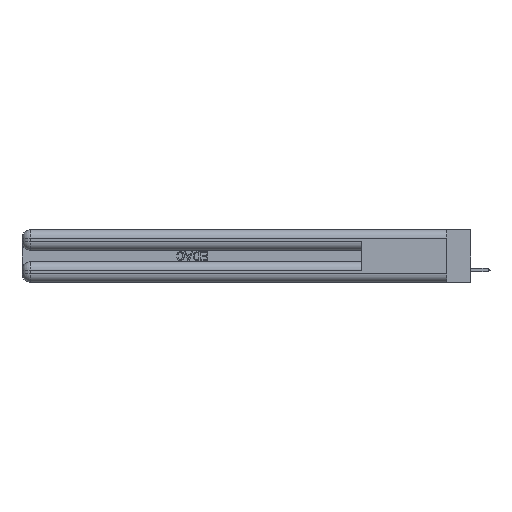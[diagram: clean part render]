
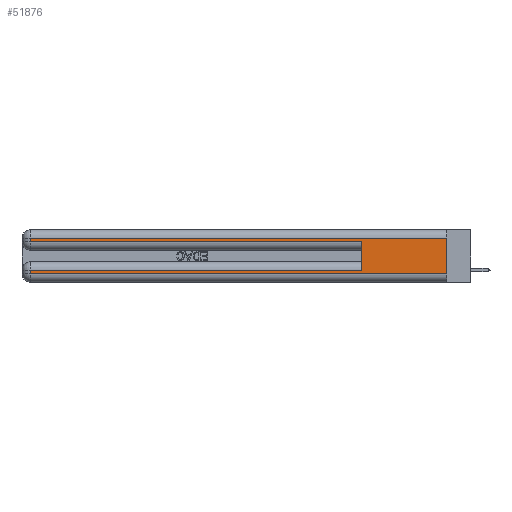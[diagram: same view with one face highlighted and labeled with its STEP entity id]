
A CAD part, left-side view. The second image highlights one B-rep face of the part: STEP entity #51876.
In plain terms, the highlighted planar face has unit normal (-1, 0, 0).
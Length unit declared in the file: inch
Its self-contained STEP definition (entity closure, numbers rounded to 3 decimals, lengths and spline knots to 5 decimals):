
#2268 = CARTESIAN_POINT ( 'NONE',  ( 0., 2.94, 0.06 ) ) ;
#2403 = DIRECTION ( 'NONE',  ( 0., 0., -1. ) ) ;
#2530 = FACE_OUTER_BOUND ( 'NONE', #23284, .T. ) ;
#3375 = VERTEX_POINT ( 'NONE', #4285 ) ;
#4037 = ORIENTED_EDGE ( 'NONE', *, *, #14851, .F. ) ;
#4285 = CARTESIAN_POINT ( 'NONE',  ( 0., 0.6, 0.085 ) ) ;
#4958 = LINE ( 'NONE', #26112, #20466 ) ;
#4983 = VERTEX_POINT ( 'NONE', #2268 ) ;
#5606 = CARTESIAN_POINT ( 'NONE',  ( 0., 0., 0.37 ) ) ;
#6268 = ORIENTED_EDGE ( 'NONE', *, *, #28849, .T. ) ;
#6938 = DIRECTION ( 'NONE',  ( 0., -1., 0. ) ) ;
#7583 = LINE ( 'NONE', #15453, #14620 ) ;
#9784 = DIRECTION ( 'NONE',  ( 0., 0., -1. ) ) ;
#9889 = AXIS2_PLACEMENT_3D ( 'NONE', #5606, #10346, #9784 ) ;
#10346 = DIRECTION ( 'NONE',  ( 1., 0., 0. ) ) ;
#10358 = DIRECTION ( 'NONE',  ( 0., -1., 0. ) ) ;
#11374 = CARTESIAN_POINT ( 'NONE',  ( 0., 0.6, 0.285 ) ) ;
#11989 = VECTOR ( 'NONE', #40810, 39.37008 ) ;
#12418 = ORIENTED_EDGE ( 'NONE', *, *, #16504, .T. ) ;
#13982 = DIRECTION ( 'NONE',  ( 0., 0., -1. ) ) ;
#14313 = CARTESIAN_POINT ( 'NONE',  ( 0., 2.94, 0.31 ) ) ;
#14620 = VECTOR ( 'NONE', #48333, 39.37008 ) ;
#14851 = EDGE_CURVE ( 'NONE', #28377, #19977, #4958, .T. ) ;
#15453 = CARTESIAN_POINT ( 'NONE',  ( 0., 0., 0.085 ) ) ;
#16504 = EDGE_CURVE ( 'NONE', #20269, #4983, #41426, .T. ) ;
#17892 = ORIENTED_EDGE ( 'NONE', *, *, #29253, .T. ) ;
#18396 = VECTOR ( 'NONE', #27814, 39.37008 ) ;
#19977 = VERTEX_POINT ( 'NONE', #35665 ) ;
#20269 = VERTEX_POINT ( 'NONE', #50969 ) ;
#20466 = VECTOR ( 'NONE', #13982, 39.37008 ) ;
#21229 = VERTEX_POINT ( 'NONE', #49828 ) ;
#22837 = LINE ( 'NONE', #41455, #11989 ) ;
#23010 = LINE ( 'NONE', #30346, #51129 ) ;
#23284 = EDGE_LOOP ( 'NONE', ( #4037, #30932, #6268, #44460, #36944, #17892, #12418, #25347 ) ) ;
#23479 = EDGE_CURVE ( 'NONE', #3375, #48098, #22837, .T. ) ;
#23999 = CARTESIAN_POINT ( 'NONE',  ( 0., 0., 0.31 ) ) ;
#25347 = ORIENTED_EDGE ( 'NONE', *, *, #35546, .T. ) ;
#26112 = CARTESIAN_POINT ( 'NONE',  ( 0., 0., 0.37 ) ) ;
#27814 = DIRECTION ( 'NONE',  ( 0., 0., -1. ) ) ;
#28377 = VERTEX_POINT ( 'NONE', #23999 ) ;
#28849 = EDGE_CURVE ( 'NONE', #40712, #21229, #23010, .T. ) ;
#29253 = EDGE_CURVE ( 'NONE', #3375, #20269, #7583, .T. ) ;
#30346 = CARTESIAN_POINT ( 'NONE',  ( 0., 2.94, 0.37 ) ) ;
#30932 = ORIENTED_EDGE ( 'NONE', *, *, #52227, .T. ) ;
#32222 = CARTESIAN_POINT ( 'NONE',  ( 0., 0., 0.31 ) ) ;
#34675 = PLANE ( 'NONE',  #9889 ) ;
#34685 = CARTESIAN_POINT ( 'NONE',  ( 0., 0., 0.06 ) ) ;
#35546 = EDGE_CURVE ( 'NONE', #4983, #19977, #46402, .T. ) ;
#35665 = CARTESIAN_POINT ( 'NONE',  ( 0., 0., 0.06 ) ) ;
#36891 = VECTOR ( 'NONE', #10358, 39.37008 ) ;
#36944 = ORIENTED_EDGE ( 'NONE', *, *, #23479, .F. ) ;
#38403 = VECTOR ( 'NONE', #6938, 39.37008 ) ;
#39519 = CARTESIAN_POINT ( 'NONE',  ( 0., 2.94, 0.37 ) ) ;
#40712 = VERTEX_POINT ( 'NONE', #14313 ) ;
#40810 = DIRECTION ( 'NONE',  ( 0., 0., 1. ) ) ;
#41426 = LINE ( 'NONE', #39519, #18396 ) ;
#41455 = CARTESIAN_POINT ( 'NONE',  ( 0., 0.6, 0.145 ) ) ;
#44200 = LINE ( 'NONE', #51841, #38403 ) ;
#44460 = ORIENTED_EDGE ( 'NONE', *, *, #47322, .T. ) ;
#46402 = LINE ( 'NONE', #34685, #36891 ) ;
#46622 = LINE ( 'NONE', #32222, #49796 ) ;
#47322 = EDGE_CURVE ( 'NONE', #21229, #48098, #44200, .T. ) ;
#48098 = VERTEX_POINT ( 'NONE', #11374 ) ;
#48333 = DIRECTION ( 'NONE',  ( 0., 1., 0. ) ) ;
#49779 = DIRECTION ( 'NONE',  ( 0., 1., 0. ) ) ;
#49796 = VECTOR ( 'NONE', #49779, 39.37008 ) ;
#49828 = CARTESIAN_POINT ( 'NONE',  ( 0., 2.94, 0.285 ) ) ;
#50969 = CARTESIAN_POINT ( 'NONE',  ( 0., 2.94, 0.085 ) ) ;
#51129 = VECTOR ( 'NONE', #2403, 39.37008 ) ;
#51841 = CARTESIAN_POINT ( 'NONE',  ( 0., 0., 0.285 ) ) ;
#51876 = ADVANCED_FACE ( 'NONE', ( #2530 ), #34675, .F. ) ;
#52227 = EDGE_CURVE ( 'NONE', #28377, #40712, #46622, .T. ) ;
